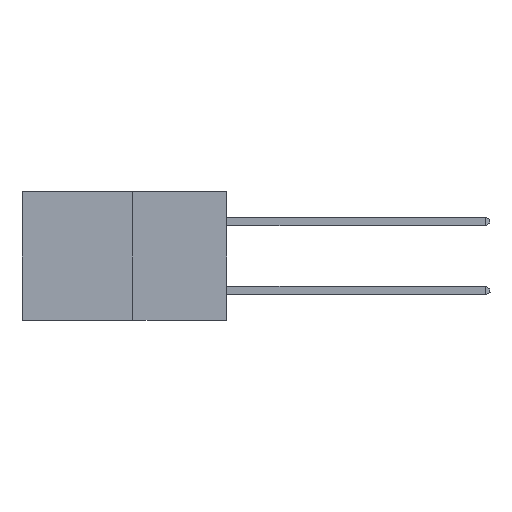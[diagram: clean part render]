
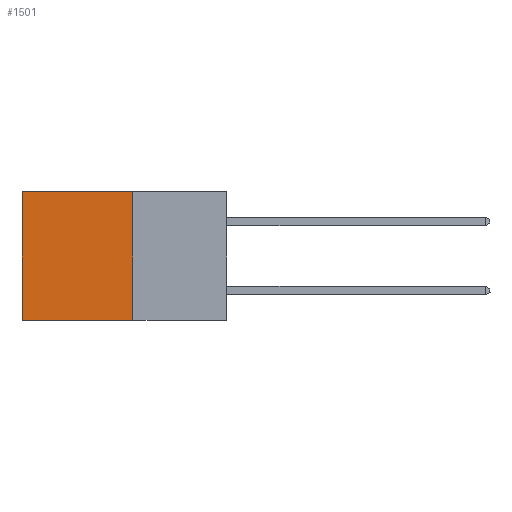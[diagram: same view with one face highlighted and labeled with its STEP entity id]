
A CAD part, left-side view. The second image highlights one B-rep face of the part: STEP entity #1501.
In plain terms, the highlighted planar face has unit normal (-1, 0, 0).
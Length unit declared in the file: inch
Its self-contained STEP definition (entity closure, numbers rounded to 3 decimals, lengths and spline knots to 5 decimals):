
#289 = CARTESIAN_POINT ( 'NONE',  ( 0.277, 0.59, -0.37 ) ) ;
#292 = EDGE_CURVE ( 'NONE', #17823, #14342, #14848, .T. ) ;
#824 = DIRECTION ( 'NONE',  ( 0., 0., -1. ) ) ;
#1318 = DIRECTION ( 'NONE',  ( 1., 0., 0. ) ) ;
#1364 = ORIENTED_EDGE ( 'NONE', *, *, #292, .T. ) ;
#1501 = ADVANCED_FACE ( 'NONE', ( #11618 ), #21955, .F. ) ;
#2369 = EDGE_CURVE ( 'NONE', #12093, #17823, #3801, .T. ) ;
#2402 = AXIS2_PLACEMENT_3D ( 'NONE', #22107, #1318, #824 ) ;
#3255 = VECTOR ( 'NONE', #4115, 39.37008 ) ;
#3801 = LINE ( 'NONE', #21119, #3255 ) ;
#4115 = DIRECTION ( 'NONE',  ( 0., 1., 0. ) ) ;
#5732 = VECTOR ( 'NONE', #14572, 39.37008 ) ;
#7806 = VECTOR ( 'NONE', #16532, 39.37008 ) ;
#9054 = EDGE_CURVE ( 'NONE', #12093, #20426, #12929, .T. ) ;
#9276 = ORIENTED_EDGE ( 'NONE', *, *, #9453, .F. ) ;
#9422 = LINE ( 'NONE', #12359, #13982 ) ;
#9453 = EDGE_CURVE ( 'NONE', #20426, #14342, #9422, .T. ) ;
#10923 = CARTESIAN_POINT ( 'NONE',  ( 0.277, 0.27, -0.37 ) ) ;
#11260 = ORIENTED_EDGE ( 'NONE', *, *, #2369, .T. ) ;
#11618 = FACE_OUTER_BOUND ( 'NONE', #18848, .T. ) ;
#12093 = VERTEX_POINT ( 'NONE', #18276 ) ;
#12359 = CARTESIAN_POINT ( 'NONE',  ( 0.277, 0.27, -0.37 ) ) ;
#12671 = ORIENTED_EDGE ( 'NONE', *, *, #9054, .F. ) ;
#12929 = LINE ( 'NONE', #18179, #7806 ) ;
#13982 = VECTOR ( 'NONE', #14059, 39.37008 ) ;
#14059 = DIRECTION ( 'NONE',  ( 0., 1., 0. ) ) ;
#14342 = VERTEX_POINT ( 'NONE', #19255 ) ;
#14572 = DIRECTION ( 'NONE',  ( 0., 0., -1. ) ) ;
#14848 = LINE ( 'NONE', #289, #5732 ) ;
#16532 = DIRECTION ( 'NONE',  ( 0., 0., -1. ) ) ;
#17823 = VERTEX_POINT ( 'NONE', #17942 ) ;
#17942 = CARTESIAN_POINT ( 'NONE',  ( 0.277, 0.59, 0. ) ) ;
#18179 = CARTESIAN_POINT ( 'NONE',  ( 0.277, 0.27, -0.37 ) ) ;
#18276 = CARTESIAN_POINT ( 'NONE',  ( 0.277, 0.27, 0. ) ) ;
#18848 = EDGE_LOOP ( 'NONE', ( #1364, #9276, #12671, #11260 ) ) ;
#19255 = CARTESIAN_POINT ( 'NONE',  ( 0.277, 0.59, -0.37 ) ) ;
#20426 = VERTEX_POINT ( 'NONE', #10923 ) ;
#21119 = CARTESIAN_POINT ( 'NONE',  ( 0.277, 0.27, 0. ) ) ;
#21955 = PLANE ( 'NONE',  #2402 ) ;
#22107 = CARTESIAN_POINT ( 'NONE',  ( 0.277, 0.27, -0.37 ) ) ;
